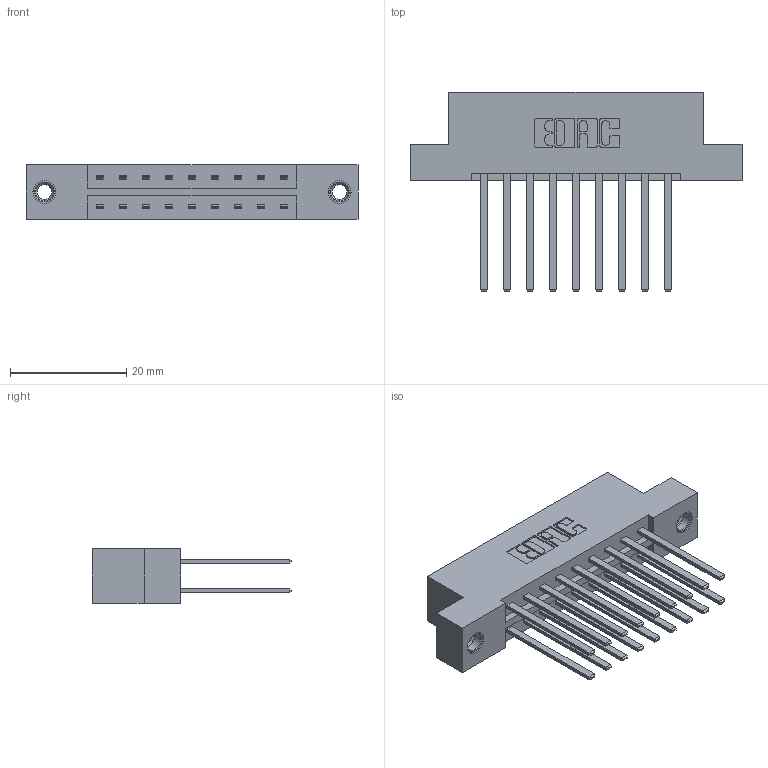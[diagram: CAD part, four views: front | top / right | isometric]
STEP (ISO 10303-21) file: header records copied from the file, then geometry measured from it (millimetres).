
FILE_DESCRIPTION (( 'STEP AP203' ), '1' );
FILE_NAME ('833-018-544-207.STEP', '2020-05-31T22:45:17', ( '' ), ( '' ), 'SwSTEP 2.0', 'SolidWorks 2020', '' );
FILE_SCHEMA (( 'CONFIG_CONTROL_DESIGN' ));
Length unit declared in the file: inch
Products named in the file (4): 345-292-001_345-293-144; 833 Part_Flush - .156 Dia - TI; 345-250-001_345-250-005-103; 833-018-544-207
Assembly tree (21 placements, depth 2):
  833-018-544-207
    833 Part_Flush - .156 Dia - TI
    345-292-001_345-293-144  x18
    345-250-001_345-250-005-103  x2
Bounding box: 57.2 x 34.3 x 9.4 mm (x, y, z)
Volume: 5770.1 mm3; surface area: 7313.6 mm2
Topology: 21 solids, 21 shells, 1002 faces, 2913 edges, 1910 vertices
Faces by surface type: plane 678, cylinder 308, cone 12, torus 4
Entity records: 11060 total; most frequent: CARTESIAN_POINT 1853, ORIENTED_EDGE 1782, DIRECTION 1669, EDGE_CURVE 891, VECTOR 747, LINE 747, VERTEX_POINT 588, AXIS2_PLACEMENT_3D 461
